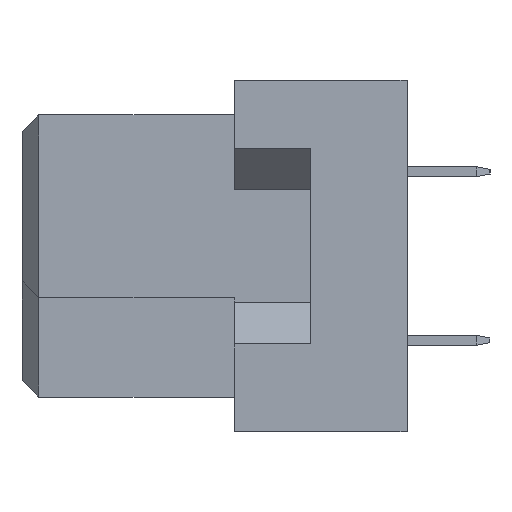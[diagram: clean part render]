
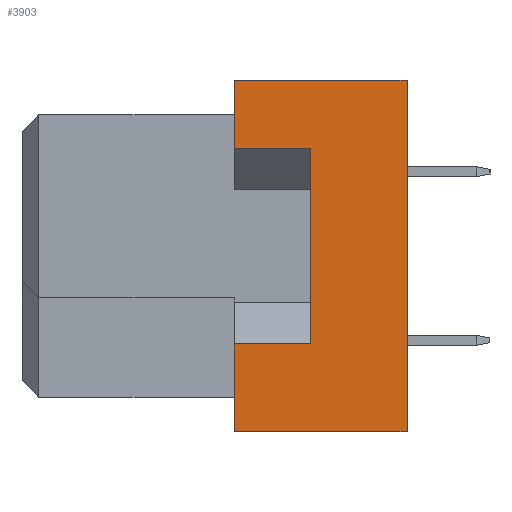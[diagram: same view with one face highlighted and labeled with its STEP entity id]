
A CAD part, left-side view. The second image highlights one B-rep face of the part: STEP entity #3903.
In plain terms, the highlighted planar face has unit normal (-1, 0, 0).
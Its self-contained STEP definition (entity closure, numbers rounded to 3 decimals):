
#67 = VERTEX_POINT ( 'NONE', #6476 ) ;
#106 = CARTESIAN_POINT ( 'NONE',  ( -27.5, -6.4, -5.3 ) ) ;
#177 = VECTOR ( 'NONE', #16091, 1000. ) ;
#735 = EDGE_CURVE ( 'NONE', #6556, #11937, #17921, .T. ) ;
#1488 = EDGE_CURVE ( 'NONE', #6556, #1508, #16583, .T. ) ;
#1508 = VERTEX_POINT ( 'NONE', #13205 ) ;
#1670 = VERTEX_POINT ( 'NONE', #17209 ) ;
#2178 = VECTOR ( 'NONE', #12972, 1000. ) ;
#2283 = PLANE ( 'NONE',  #17708 ) ;
#2496 = CARTESIAN_POINT ( 'NONE',  ( -27.5, -11.6, 5.3 ) ) ;
#3448 = DIRECTION ( 'NONE',  ( 0., 0., 1. ) ) ;
#3903 = ADVANCED_FACE ( 'NONE', ( #7025 ), #2283, .T. ) ;
#4367 = LINE ( 'NONE', #18574, #4557 ) ;
#4557 = VECTOR ( 'NONE', #4587, 1000. ) ;
#4587 = DIRECTION ( 'NONE',  ( 0., 0., 1. ) ) ;
#4820 = CARTESIAN_POINT ( 'NONE',  ( -27.5, -8.7, -2.65 ) ) ;
#4828 = LINE ( 'NONE', #12823, #17148 ) ;
#5058 = CARTESIAN_POINT ( 'NONE',  ( -27.5, -11.6, 5.3 ) ) ;
#5359 = LINE ( 'NONE', #5058, #18040 ) ;
#6260 = EDGE_LOOP ( 'NONE', ( #12327, #14469, #11342, #17421, #17286, #8079, #15977, #17490 ) ) ;
#6476 = CARTESIAN_POINT ( 'NONE',  ( -27.5, -6.4, 3.25 ) ) ;
#6530 = DIRECTION ( 'NONE',  ( 0., 0., 1. ) ) ;
#6556 = VERTEX_POINT ( 'NONE', #11699 ) ;
#7025 = FACE_OUTER_BOUND ( 'NONE', #6260, .T. ) ;
#7339 = DIRECTION ( 'NONE',  ( 0., 0., 1. ) ) ;
#7614 = CARTESIAN_POINT ( 'NONE',  ( -27.5, -8.7, -2.65 ) ) ;
#8079 = ORIENTED_EDGE ( 'NONE', *, *, #19335, .F. ) ;
#9158 = EDGE_CURVE ( 'NONE', #11937, #12595, #17663, .T. ) ;
#9929 = CARTESIAN_POINT ( 'NONE',  ( -27.5, -11.6, -5.3 ) ) ;
#10367 = EDGE_CURVE ( 'NONE', #1670, #67, #4828, .T. ) ;
#10374 = CARTESIAN_POINT ( 'NONE',  ( -27.5, -6.4, -2.65 ) ) ;
#11342 = ORIENTED_EDGE ( 'NONE', *, *, #735, .F. ) ;
#11566 = VERTEX_POINT ( 'NONE', #18641 ) ;
#11699 = CARTESIAN_POINT ( 'NONE',  ( -27.5, -11.6, -5.3 ) ) ;
#11715 = VECTOR ( 'NONE', #3448, 1000. ) ;
#11937 = VERTEX_POINT ( 'NONE', #18507 ) ;
#12327 = ORIENTED_EDGE ( 'NONE', *, *, #16753, .T. ) ;
#12595 = VERTEX_POINT ( 'NONE', #10374 ) ;
#12713 = LINE ( 'NONE', #4820, #177 ) ;
#12714 = CARTESIAN_POINT ( 'NONE',  ( -27.5, -6.4, -5.3 ) ) ;
#12823 = CARTESIAN_POINT ( 'NONE',  ( -27.5, -8.7, 3.25 ) ) ;
#12972 = DIRECTION ( 'NONE',  ( 0., 1., 0. ) ) ;
#13205 = CARTESIAN_POINT ( 'NONE',  ( -27.5, -11.6, 5.3 ) ) ;
#13445 = DIRECTION ( 'NONE',  ( -1., 0., 0. ) ) ;
#14469 = ORIENTED_EDGE ( 'NONE', *, *, #9158, .F. ) ;
#14534 = LINE ( 'NONE', #106, #19021 ) ;
#14816 = DIRECTION ( 'NONE',  ( 0., 1., 0. ) ) ;
#15977 = ORIENTED_EDGE ( 'NONE', *, *, #10367, .F. ) ;
#16091 = DIRECTION ( 'NONE',  ( 0., 1., 0. ) ) ;
#16583 = LINE ( 'NONE', #17850, #18050 ) ;
#16753 = EDGE_CURVE ( 'NONE', #18731, #12595, #12713, .T. ) ;
#17017 = EDGE_CURVE ( 'NONE', #18731, #1670, #4367, .T. ) ;
#17148 = VECTOR ( 'NONE', #14816, 1000. ) ;
#17209 = CARTESIAN_POINT ( 'NONE',  ( -27.5, -8.7, 3.25 ) ) ;
#17286 = ORIENTED_EDGE ( 'NONE', *, *, #18174, .T. ) ;
#17421 = ORIENTED_EDGE ( 'NONE', *, *, #1488, .T. ) ;
#17490 = ORIENTED_EDGE ( 'NONE', *, *, #17017, .F. ) ;
#17663 = LINE ( 'NONE', #12714, #11715 ) ;
#17708 = AXIS2_PLACEMENT_3D ( 'NONE', #2496, #13445, #7339 ) ;
#17850 = CARTESIAN_POINT ( 'NONE',  ( -27.5, -11.6, 5.3 ) ) ;
#17921 = LINE ( 'NONE', #9929, #2178 ) ;
#18040 = VECTOR ( 'NONE', #18196, 1000. ) ;
#18050 = VECTOR ( 'NONE', #19730, 1000. ) ;
#18174 = EDGE_CURVE ( 'NONE', #1508, #11566, #5359, .T. ) ;
#18196 = DIRECTION ( 'NONE',  ( 0., 1., 0. ) ) ;
#18507 = CARTESIAN_POINT ( 'NONE',  ( -27.5, -6.4, -5.3 ) ) ;
#18574 = CARTESIAN_POINT ( 'NONE',  ( -27.5, -8.7, -2.65 ) ) ;
#18641 = CARTESIAN_POINT ( 'NONE',  ( -27.5, -6.4, 5.3 ) ) ;
#18731 = VERTEX_POINT ( 'NONE', #7614 ) ;
#19021 = VECTOR ( 'NONE', #6530, 1000. ) ;
#19335 = EDGE_CURVE ( 'NONE', #67, #11566, #14534, .T. ) ;
#19730 = DIRECTION ( 'NONE',  ( 0., 0., 1. ) ) ;
